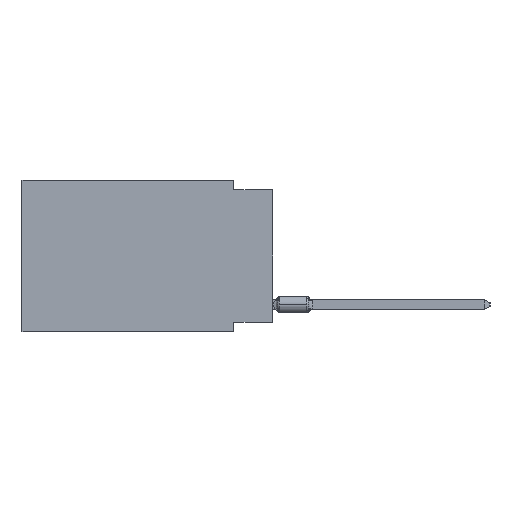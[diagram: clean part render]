
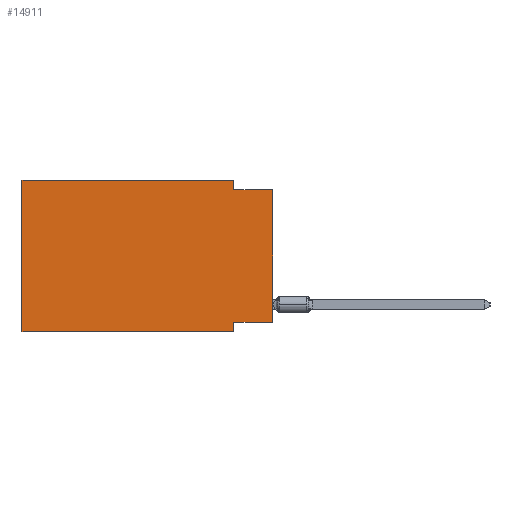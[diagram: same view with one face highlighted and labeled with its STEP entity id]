
A CAD part, left-side view. The second image highlights one B-rep face of the part: STEP entity #14911.
In plain terms, the highlighted planar face has unit normal (-1, 0, 0).
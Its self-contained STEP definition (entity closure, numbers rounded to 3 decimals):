
#220 = AXIS2_PLACEMENT_3D ( 'NONE', #28895, #19307, #29240 ) ;
#3251 = CARTESIAN_POINT ( 'NONE',  ( 0., 16.383, -9.906 ) ) ;
#4647 = ORIENTED_EDGE ( 'NONE', *, *, #61893, .F. ) ;
#5604 = LINE ( 'NONE', #11719, #54285 ) ;
#6717 = VERTEX_POINT ( 'NONE', #6838 ) ;
#6838 = CARTESIAN_POINT ( 'NONE',  ( 0., 2.54, -9.271 ) ) ;
#9822 = CARTESIAN_POINT ( 'NONE',  ( 0., 2.54, 0. ) ) ;
#10119 = CARTESIAN_POINT ( 'NONE',  ( 0., 2.54, -0.635 ) ) ;
#10151 = CARTESIAN_POINT ( 'NONE',  ( 0., 16.383, 0. ) ) ;
#10805 = DIRECTION ( 'NONE',  ( 0., -1., 0. ) ) ;
#11404 = ORIENTED_EDGE ( 'NONE', *, *, #64027, .F. ) ;
#11719 = CARTESIAN_POINT ( 'NONE',  ( 0., 2.54, 0. ) ) ;
#11750 = CARTESIAN_POINT ( 'NONE',  ( 0., 16.383, -9.906 ) ) ;
#13549 = EDGE_CURVE ( 'NONE', #16115, #34593, #61166, .T. ) ;
#14704 = CARTESIAN_POINT ( 'NONE',  ( 0., 2.54, -9.906 ) ) ;
#14911 = ADVANCED_FACE ( 'NONE', ( #24438 ), #43932, .F. ) ;
#15365 = CARTESIAN_POINT ( 'NONE',  ( 0., 0., -9.271 ) ) ;
#15639 = EDGE_CURVE ( 'NONE', #6717, #57017, #43114, .T. ) ;
#15824 = EDGE_CURVE ( 'NONE', #63857, #28538, #23938, .T. ) ;
#16115 = VERTEX_POINT ( 'NONE', #15365 ) ;
#18809 = VECTOR ( 'NONE', #33192, 1000. ) ;
#19307 = DIRECTION ( 'NONE',  ( 1., 0., 0. ) ) ;
#20780 = DIRECTION ( 'NONE',  ( 0., 1., 0. ) ) ;
#21347 = DIRECTION ( 'NONE',  ( 0., -1., 0. ) ) ;
#22916 = VECTOR ( 'NONE', #33872, 1000. ) ;
#23307 = CARTESIAN_POINT ( 'NONE',  ( 0., 0., -0.635 ) ) ;
#23938 = LINE ( 'NONE', #64615, #18809 ) ;
#24438 = FACE_OUTER_BOUND ( 'NONE', #60071, .T. ) ;
#25403 = ORIENTED_EDGE ( 'NONE', *, *, #64817, .F. ) ;
#26011 = EDGE_CURVE ( 'NONE', #50452, #34593, #65268, .T. ) ;
#26561 = VERTEX_POINT ( 'NONE', #9822 ) ;
#28489 = ORIENTED_EDGE ( 'NONE', *, *, #55078, .T. ) ;
#28538 = VERTEX_POINT ( 'NONE', #51831 ) ;
#28895 = CARTESIAN_POINT ( 'NONE',  ( 0., 16.383, 0. ) ) ;
#29065 = CARTESIAN_POINT ( 'NONE',  ( 0., 0., -0.635 ) ) ;
#29240 = DIRECTION ( 'NONE',  ( 0., 0., -1. ) ) ;
#29741 = VECTOR ( 'NONE', #62585, 1000. ) ;
#31715 = CARTESIAN_POINT ( 'NONE',  ( 0., 0., -9.271 ) ) ;
#32400 = VECTOR ( 'NONE', #20780, 1000. ) ;
#33192 = DIRECTION ( 'NONE',  ( 0., 0., 1. ) ) ;
#33872 = DIRECTION ( 'NONE',  ( 0., 0., 1. ) ) ;
#34593 = VERTEX_POINT ( 'NONE', #23307 ) ;
#35300 = VECTOR ( 'NONE', #49575, 1000. ) ;
#35911 = ORIENTED_EDGE ( 'NONE', *, *, #15824, .F. ) ;
#37307 = CARTESIAN_POINT ( 'NONE',  ( 0., 2.54, -9.906 ) ) ;
#41361 = ORIENTED_EDGE ( 'NONE', *, *, #26011, .F. ) ;
#43114 = LINE ( 'NONE', #37307, #29741 ) ;
#43932 = PLANE ( 'NONE',  #220 ) ;
#44214 = ORIENTED_EDGE ( 'NONE', *, *, #15639, .F. ) ;
#46080 = LINE ( 'NONE', #31715, #32400 ) ;
#47895 = VECTOR ( 'NONE', #10805, 1000. ) ;
#48297 = DIRECTION ( 'NONE',  ( 0., 0., -1. ) ) ;
#49575 = DIRECTION ( 'NONE',  ( 0., -1., 0. ) ) ;
#50452 = VERTEX_POINT ( 'NONE', #10119 ) ;
#51831 = CARTESIAN_POINT ( 'NONE',  ( 0., 16.383, 0. ) ) ;
#53460 = LINE ( 'NONE', #11750, #61233 ) ;
#54285 = VECTOR ( 'NONE', #48297, 1000. ) ;
#54379 = CARTESIAN_POINT ( 'NONE',  ( 0., 0., 0. ) ) ;
#55078 = EDGE_CURVE ( 'NONE', #63857, #57017, #53460, .T. ) ;
#57017 = VERTEX_POINT ( 'NONE', #14704 ) ;
#57622 = LINE ( 'NONE', #10151, #47895 ) ;
#60071 = EDGE_LOOP ( 'NONE', ( #60209, #41361, #11404, #25403, #35911, #28489, #44214, #4647 ) ) ;
#60209 = ORIENTED_EDGE ( 'NONE', *, *, #13549, .T. ) ;
#61166 = LINE ( 'NONE', #54379, #22916 ) ;
#61233 = VECTOR ( 'NONE', #21347, 1000. ) ;
#61893 = EDGE_CURVE ( 'NONE', #16115, #6717, #46080, .T. ) ;
#62585 = DIRECTION ( 'NONE',  ( 0., 0., -1. ) ) ;
#63857 = VERTEX_POINT ( 'NONE', #3251 ) ;
#64027 = EDGE_CURVE ( 'NONE', #26561, #50452, #5604, .T. ) ;
#64615 = CARTESIAN_POINT ( 'NONE',  ( 0., 16.383, 0. ) ) ;
#64817 = EDGE_CURVE ( 'NONE', #28538, #26561, #57622, .T. ) ;
#65268 = LINE ( 'NONE', #29065, #35300 ) ;
